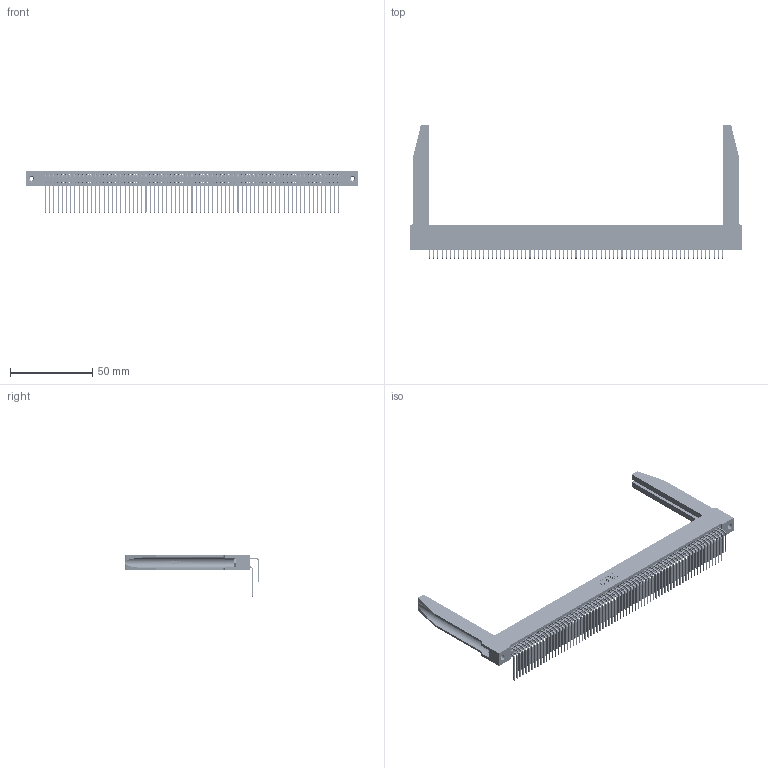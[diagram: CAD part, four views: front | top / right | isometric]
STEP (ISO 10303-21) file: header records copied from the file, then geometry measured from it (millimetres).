
FILE_DESCRIPTION (( 'STEP AP203' ), '1' );
FILE_NAME ('345-142-559-278.STEP', '2019-11-09T05:39:42', ( '' ), ( '' ), 'SwSTEP 2.0', 'SolidWorks 2016', '' );
FILE_SCHEMA (( 'CONFIG_CONTROL_DESIGN' ));
Length unit declared in the file: inch
Products named in the file (6): 345-292-001_559 Tail - 2; 345-220-078_345-220-078; 345 Part_Flush Mounting Lugs - 0.156 Dia-TH; 345-142-559-278; 345-292-001_558 559 Tail - 1; 345-250-001_345-250-001-102
Assembly tree (147 placements, depth 2):
  345-142-559-278
    345 Part_Flush Mounting Lugs - 0.156 Dia-TH
    345-292-001_558 559 Tail - 1  x71
    345-292-001_559 Tail - 2  x71
    345-250-001_345-250-001-102  x2
    345-220-078_345-220-078  x2
Bounding box: 201.57 x 81.52 x 25.53 mm (x, y, z)
Volume: 28439.9 mm3; surface area: 41805.1 mm2
Topology: 147 solids, 147 shells, 7744 faces, 22959 edges, 15106 vertices
Faces by surface type: plane 5192, cylinder 2500, bspline 36, cone 12, torus 4
Entity records: 58196 total; most frequent: CARTESIAN_POINT 10690, ORIENTED_EDGE 9470, DIRECTION 8357, EDGE_CURVE 4735, LINE 4185, VECTOR 4185, VERTEX_POINT 3148, AXIS2_PLACEMENT_3D 2086
